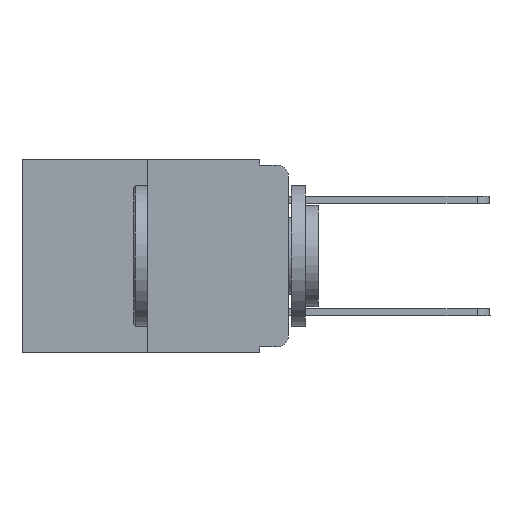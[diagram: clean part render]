
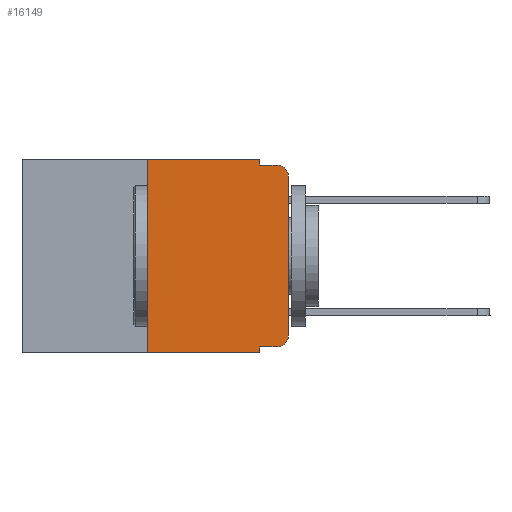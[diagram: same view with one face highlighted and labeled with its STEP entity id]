
A CAD part, left-side view. The second image highlights one B-rep face of the part: STEP entity #16149.
In plain terms, the highlighted planar face has unit normal (-1, 0, 0).
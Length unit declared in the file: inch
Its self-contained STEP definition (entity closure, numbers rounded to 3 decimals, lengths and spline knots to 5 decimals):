
#662 = CARTESIAN_POINT ( 'NONE',  ( 0., 0.051, -0.343 ) ) ;
#1205 = EDGE_CURVE ( 'NONE', #16457, #21657, #24258, .T. ) ;
#1656 = ORIENTED_EDGE ( 'NONE', *, *, #22914, .T. ) ;
#1696 = DIRECTION ( 'NONE',  ( 0., 0., -1. ) ) ;
#2410 = VERTEX_POINT ( 'NONE', #662 ) ;
#2526 = VERTEX_POINT ( 'NONE', #7045 ) ;
#2596 = DIRECTION ( 'NONE',  ( 0., 0., 1. ) ) ;
#2942 = CARTESIAN_POINT ( 'NONE',  ( 0., 0.051, -0.333 ) ) ;
#3436 = LINE ( 'NONE', #7788, #25023 ) ;
#3441 = AXIS2_PLACEMENT_3D ( 'NONE', #22075, #22559, #10499 ) ;
#3853 = VECTOR ( 'NONE', #9315, 39.37008 ) ;
#3921 = EDGE_CURVE ( 'NONE', #16212, #6812, #9250, .T. ) ;
#3990 = CARTESIAN_POINT ( 'NONE',  ( 0., 0.051, 0. ) ) ;
#4764 = LINE ( 'NONE', #20571, #15835 ) ;
#4997 = DIRECTION ( 'NONE',  ( 0., 0., -1. ) ) ;
#5037 = ORIENTED_EDGE ( 'NONE', *, *, #3921, .F. ) ;
#5268 = CARTESIAN_POINT ( 'NONE',  ( 0., 0.051, 0. ) ) ;
#6233 = VECTOR ( 'NONE', #9510, 39.37008 ) ;
#6559 = LINE ( 'NONE', #24037, #9942 ) ;
#6658 = CARTESIAN_POINT ( 'NONE',  ( 0., 0.051, -0.333 ) ) ;
#6812 = VERTEX_POINT ( 'NONE', #14756 ) ;
#7045 = CARTESIAN_POINT ( 'NONE',  ( 0., 0.25, -0.343 ) ) ;
#7527 = VERTEX_POINT ( 'NONE', #13912 ) ;
#7788 = CARTESIAN_POINT ( 'NONE',  ( 0., 0.051, 0. ) ) ;
#8013 = ORIENTED_EDGE ( 'NONE', *, *, #12404, .F. ) ;
#8642 = VECTOR ( 'NONE', #4997, 39.37008 ) ;
#9034 = CARTESIAN_POINT ( 'NONE',  ( 0., 0., -0.03 ) ) ;
#9250 = LINE ( 'NONE', #5268, #8642 ) ;
#9315 = DIRECTION ( 'NONE',  ( 0., -1., 0. ) ) ;
#9510 = DIRECTION ( 'NONE',  ( 0., -1., 0. ) ) ;
#9543 = EDGE_LOOP ( 'NONE', ( #14028, #1656, #12808, #5037, #10529, #10120, #20976, #8013, #12063, #14009 ) ) ;
#9942 = VECTOR ( 'NONE', #2596, 39.37008 ) ;
#10120 = ORIENTED_EDGE ( 'NONE', *, *, #19963, .F. ) ;
#10499 = DIRECTION ( 'NONE',  ( 0., 0., -1. ) ) ;
#10529 = ORIENTED_EDGE ( 'NONE', *, *, #18016, .F. ) ;
#10977 = CARTESIAN_POINT ( 'NONE',  ( 0., 0., -0.313 ) ) ;
#11349 = CARTESIAN_POINT ( 'NONE',  ( 0., 0.02, -0.313 ) ) ;
#11442 = DIRECTION ( 'NONE',  ( 1., 0., 0. ) ) ;
#12063 = ORIENTED_EDGE ( 'NONE', *, *, #1205, .T. ) ;
#12404 = EDGE_CURVE ( 'NONE', #16457, #2410, #3436, .T. ) ;
#12594 = DIRECTION ( 'NONE',  ( 0., 0., 1. ) ) ;
#12808 = ORIENTED_EDGE ( 'NONE', *, *, #16164, .F. ) ;
#13072 = VERTEX_POINT ( 'NONE', #20487 ) ;
#13128 = EDGE_CURVE ( 'NONE', #21657, #24790, #14768, .T. ) ;
#13546 = DIRECTION ( 'NONE',  ( 0., -1., 0. ) ) ;
#13912 = CARTESIAN_POINT ( 'NONE',  ( 0., 0.02, -0.01 ) ) ;
#14009 = ORIENTED_EDGE ( 'NONE', *, *, #13128, .T. ) ;
#14028 = ORIENTED_EDGE ( 'NONE', *, *, #14645, .T. ) ;
#14497 = DIRECTION ( 'NONE',  ( 0., -1., 0. ) ) ;
#14645 = EDGE_CURVE ( 'NONE', #24790, #24829, #6559, .T. ) ;
#14756 = CARTESIAN_POINT ( 'NONE',  ( 0., 0.051, -0.01 ) ) ;
#14768 = CIRCLE ( 'NONE', #16395, 0.02 ) ;
#15294 = FACE_OUTER_BOUND ( 'NONE', #9543, .T. ) ;
#15791 = LINE ( 'NONE', #23643, #6233 ) ;
#15835 = VECTOR ( 'NONE', #12594, 39.37008 ) ;
#16149 = ADVANCED_FACE ( 'NONE', ( #15294 ), #19281, .F. ) ;
#16164 = EDGE_CURVE ( 'NONE', #6812, #7527, #15791, .T. ) ;
#16212 = VERTEX_POINT ( 'NONE', #3990 ) ;
#16395 = AXIS2_PLACEMENT_3D ( 'NONE', #11349, #23670, #21123 ) ;
#16457 = VERTEX_POINT ( 'NONE', #2942 ) ;
#17172 = DIRECTION ( 'NONE',  ( 0., 0., -1. ) ) ;
#18016 = EDGE_CURVE ( 'NONE', #13072, #16212, #23056, .T. ) ;
#19281 = PLANE ( 'NONE',  #20209 ) ;
#19349 = LINE ( 'NONE', #23822, #19869 ) ;
#19443 = CIRCLE ( 'NONE', #3441, 0.02 ) ;
#19869 = VECTOR ( 'NONE', #13546, 39.37008 ) ;
#19963 = EDGE_CURVE ( 'NONE', #2526, #13072, #4764, .T. ) ;
#20209 = AXIS2_PLACEMENT_3D ( 'NONE', #21347, #11442, #1696 ) ;
#20487 = CARTESIAN_POINT ( 'NONE',  ( 0., 0.25, 0. ) ) ;
#20571 = CARTESIAN_POINT ( 'NONE',  ( 0., 0.25, 0. ) ) ;
#20976 = ORIENTED_EDGE ( 'NONE', *, *, #23199, .T. ) ;
#21123 = DIRECTION ( 'NONE',  ( 0., 0., -1. ) ) ;
#21347 = CARTESIAN_POINT ( 'NONE',  ( 0., 0.473, 0. ) ) ;
#21657 = VERTEX_POINT ( 'NONE', #22555 ) ;
#22075 = CARTESIAN_POINT ( 'NONE',  ( 0., 0.02, -0.03 ) ) ;
#22555 = CARTESIAN_POINT ( 'NONE',  ( 0., 0.02, -0.333 ) ) ;
#22559 = DIRECTION ( 'NONE',  ( -1., 0., 0. ) ) ;
#22914 = EDGE_CURVE ( 'NONE', #24829, #7527, #19443, .T. ) ;
#23056 = LINE ( 'NONE', #23713, #3853 ) ;
#23199 = EDGE_CURVE ( 'NONE', #2526, #2410, #19349, .T. ) ;
#23571 = VECTOR ( 'NONE', #14497, 39.37008 ) ;
#23643 = CARTESIAN_POINT ( 'NONE',  ( 0., 0.051, -0.01 ) ) ;
#23670 = DIRECTION ( 'NONE',  ( -1., 0., 0. ) ) ;
#23713 = CARTESIAN_POINT ( 'NONE',  ( 0., 0.473, 0. ) ) ;
#23822 = CARTESIAN_POINT ( 'NONE',  ( 0., 0.473, -0.343 ) ) ;
#24037 = CARTESIAN_POINT ( 'NONE',  ( 0., 0., 0. ) ) ;
#24258 = LINE ( 'NONE', #6658, #23571 ) ;
#24790 = VERTEX_POINT ( 'NONE', #10977 ) ;
#24829 = VERTEX_POINT ( 'NONE', #9034 ) ;
#25023 = VECTOR ( 'NONE', #17172, 39.37008 ) ;
